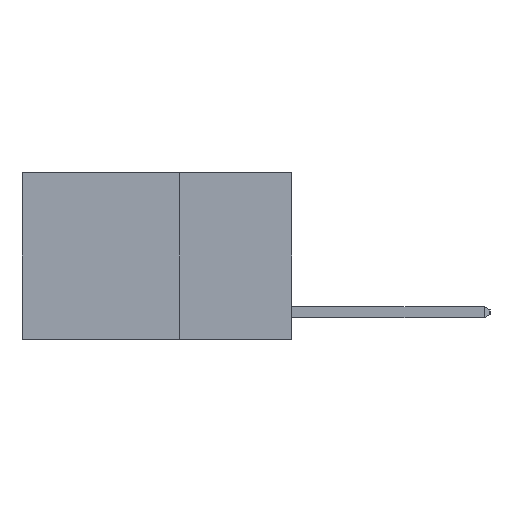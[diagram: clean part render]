
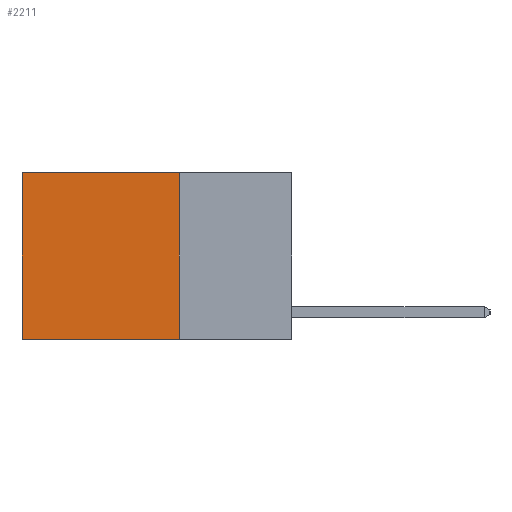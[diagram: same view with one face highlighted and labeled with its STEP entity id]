
A CAD part, left-side view. The second image highlights one B-rep face of the part: STEP entity #2211.
In plain terms, the highlighted planar face has unit normal (-1, 0, 0).
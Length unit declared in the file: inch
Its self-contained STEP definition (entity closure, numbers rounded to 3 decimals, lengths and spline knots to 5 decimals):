
#96 = DIRECTION ( 'NONE',  ( 0., 1., 0. ) ) ;
#1334 = VECTOR ( 'NONE', #2188, 39.37008 ) ;
#1338 = VERTEX_POINT ( 'NONE', #1998 ) ;
#1731 = VERTEX_POINT ( 'NONE', #8778 ) ;
#1998 = CARTESIAN_POINT ( 'NONE',  ( 0.2625, 0.25, -0.37 ) ) ;
#2078 = VERTEX_POINT ( 'NONE', #7940 ) ;
#2188 = DIRECTION ( 'NONE',  ( 0., 0., -1. ) ) ;
#2211 = ADVANCED_FACE ( 'NONE', ( #3296 ), #8954, .F. ) ;
#2604 = AXIS2_PLACEMENT_3D ( 'NONE', #8989, #8883, #8873 ) ;
#2664 = DIRECTION ( 'NONE',  ( 0., 1., 0. ) ) ;
#2879 = VECTOR ( 'NONE', #96, 39.37008 ) ;
#2937 = CARTESIAN_POINT ( 'NONE',  ( 0.2625, 0.25, 0. ) ) ;
#3296 = FACE_OUTER_BOUND ( 'NONE', #5634, .T. ) ;
#3323 = ORIENTED_EDGE ( 'NONE', *, *, #7500, .F. ) ;
#4017 = CARTESIAN_POINT ( 'NONE',  ( 0.2625, 0.6, -0.37 ) ) ;
#4098 = ORIENTED_EDGE ( 'NONE', *, *, #5835, .T. ) ;
#4102 = CARTESIAN_POINT ( 'NONE',  ( 0.2625, 0.25, -0.37 ) ) ;
#4325 = ORIENTED_EDGE ( 'NONE', *, *, #6324, .F. ) ;
#4768 = LINE ( 'NONE', #6440, #2879 ) ;
#4963 = VECTOR ( 'NONE', #6000, 39.37008 ) ;
#5334 = CARTESIAN_POINT ( 'NONE',  ( 0.2625, 0.6, 0. ) ) ;
#5453 = ORIENTED_EDGE ( 'NONE', *, *, #6965, .T. ) ;
#5634 = EDGE_LOOP ( 'NONE', ( #5453, #4325, #3323, #4098 ) ) ;
#5835 = EDGE_CURVE ( 'NONE', #2078, #1731, #4768, .T. ) ;
#6000 = DIRECTION ( 'NONE',  ( 0., 0., -1. ) ) ;
#6161 = VERTEX_POINT ( 'NONE', #4017 ) ;
#6324 = EDGE_CURVE ( 'NONE', #1338, #6161, #7405, .T. ) ;
#6440 = CARTESIAN_POINT ( 'NONE',  ( 0.2625, 0.25, 0. ) ) ;
#6949 = LINE ( 'NONE', #2937, #1334 ) ;
#6965 = EDGE_CURVE ( 'NONE', #1731, #6161, #8587, .T. ) ;
#7180 = VECTOR ( 'NONE', #2664, 39.37008 ) ;
#7405 = LINE ( 'NONE', #4102, #7180 ) ;
#7500 = EDGE_CURVE ( 'NONE', #2078, #1338, #6949, .T. ) ;
#7940 = CARTESIAN_POINT ( 'NONE',  ( 0.2625, 0.25, 0. ) ) ;
#8587 = LINE ( 'NONE', #5334, #4963 ) ;
#8778 = CARTESIAN_POINT ( 'NONE',  ( 0.2625, 0.6, 0. ) ) ;
#8873 = DIRECTION ( 'NONE',  ( 0., 0., -1. ) ) ;
#8883 = DIRECTION ( 'NONE',  ( 1., 0., 0. ) ) ;
#8954 = PLANE ( 'NONE',  #2604 ) ;
#8989 = CARTESIAN_POINT ( 'NONE',  ( 0.2625, 0.25, 0. ) ) ;
